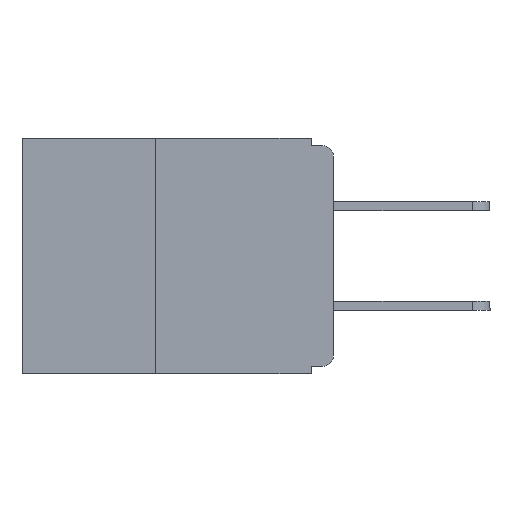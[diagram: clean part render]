
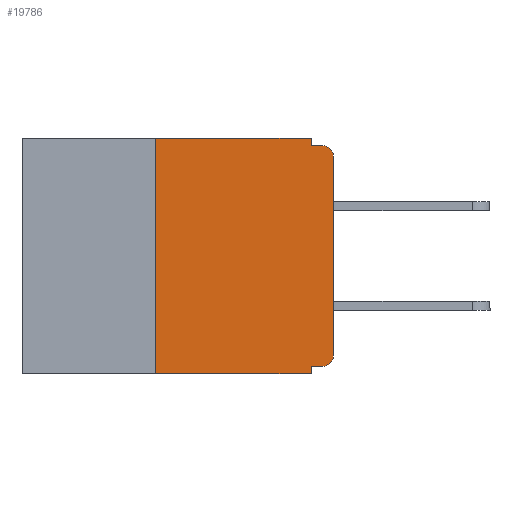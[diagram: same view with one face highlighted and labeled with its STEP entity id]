
A CAD part, left-side view. The second image highlights one B-rep face of the part: STEP entity #19786.
In plain terms, the highlighted planar face has unit normal (-1, 0, 0).
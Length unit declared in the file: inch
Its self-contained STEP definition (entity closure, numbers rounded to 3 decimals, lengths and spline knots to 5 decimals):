
#32 = CARTESIAN_POINT ( 'NONE',  ( 0., 0.031, -0.33 ) ) ;
#624 = VERTEX_POINT ( 'NONE', #32 ) ;
#645 = VERTEX_POINT ( 'NONE', #4479 ) ;
#825 = CARTESIAN_POINT ( 'NONE',  ( 0., 0.031, 0. ) ) ;
#1121 = VECTOR ( 'NONE', #8629, 39.37008 ) ;
#1186 = DIRECTION ( 'NONE',  ( 0., 0., 1. ) ) ;
#1564 = EDGE_CURVE ( 'NONE', #7581, #8345, #25323, .T. ) ;
#2440 = CARTESIAN_POINT ( 'NONE',  ( 0., 0., -0.01 ) ) ;
#2528 = ORIENTED_EDGE ( 'NONE', *, *, #4755, .T. ) ;
#3436 = LINE ( 'NONE', #8427, #21865 ) ;
#3734 = CIRCLE ( 'NONE', #17388, 0.015 ) ;
#4479 = CARTESIAN_POINT ( 'NONE',  ( 0., 0.25, -0.33 ) ) ;
#4483 = VERTEX_POINT ( 'NONE', #14346 ) ;
#4755 = EDGE_CURVE ( 'NONE', #22845, #7918, #9734, .T. ) ;
#4985 = DIRECTION ( 'NONE',  ( 0., -1., 0. ) ) ;
#6077 = VERTEX_POINT ( 'NONE', #9265 ) ;
#6265 = LINE ( 'NONE', #22654, #18276 ) ;
#7231 = CARTESIAN_POINT ( 'NONE',  ( 0., 0.015, -0.305 ) ) ;
#7581 = VERTEX_POINT ( 'NONE', #825 ) ;
#7740 = LINE ( 'NONE', #25043, #1121 ) ;
#7918 = VERTEX_POINT ( 'NONE', #28722 ) ;
#7936 = VECTOR ( 'NONE', #21931, 39.37008 ) ;
#8121 = ORIENTED_EDGE ( 'NONE', *, *, #26197, .T. ) ;
#8345 = VERTEX_POINT ( 'NONE', #16468 ) ;
#8427 = CARTESIAN_POINT ( 'NONE',  ( 0., 0., 0. ) ) ;
#8629 = DIRECTION ( 'NONE',  ( 0., -1., 0. ) ) ;
#9265 = CARTESIAN_POINT ( 'NONE',  ( 0., 0.031, -0.32 ) ) ;
#9291 = DIRECTION ( 'NONE',  ( 0., 1., 0. ) ) ;
#9700 = EDGE_CURVE ( 'NONE', #29924, #6077, #18430, .T. ) ;
#9725 = DIRECTION ( 'NONE',  ( 0., 0., -1. ) ) ;
#9734 = CIRCLE ( 'NONE', #17256, 0.015 ) ;
#9799 = CARTESIAN_POINT ( 'NONE',  ( 0., 0., -0.025 ) ) ;
#10445 = DIRECTION ( 'NONE',  ( 1., 0., 0. ) ) ;
#12741 = PLANE ( 'NONE',  #28231 ) ;
#14346 = CARTESIAN_POINT ( 'NONE',  ( 0., 0., -0.305 ) ) ;
#14945 = CARTESIAN_POINT ( 'NONE',  ( 0., 0.015, -0.32 ) ) ;
#15527 = DIRECTION ( 'NONE',  ( 0., 0., -1. ) ) ;
#15564 = DIRECTION ( 'NONE',  ( -1., 0., 0. ) ) ;
#15956 = CARTESIAN_POINT ( 'NONE',  ( 0., 0.015, -0.025 ) ) ;
#16377 = CARTESIAN_POINT ( 'NONE',  ( 0., 0., -0.32 ) ) ;
#16468 = CARTESIAN_POINT ( 'NONE',  ( 0., 0.031, -0.01 ) ) ;
#16560 = CARTESIAN_POINT ( 'NONE',  ( 0., 0.25, 0. ) ) ;
#16858 = ORIENTED_EDGE ( 'NONE', *, *, #17650, .F. ) ;
#16893 = EDGE_LOOP ( 'NONE', ( #18724, #2528, #16858, #24635, #30040, #24900, #8121, #21012, #29173, #21923 ) ) ;
#17256 = AXIS2_PLACEMENT_3D ( 'NONE', #15956, #15564, #15527 ) ;
#17388 = AXIS2_PLACEMENT_3D ( 'NONE', #7231, #23844, #9725 ) ;
#17467 = FACE_OUTER_BOUND ( 'NONE', #16893, .T. ) ;
#17650 = EDGE_CURVE ( 'NONE', #8345, #7918, #19851, .T. ) ;
#18276 = VECTOR ( 'NONE', #24957, 39.37008 ) ;
#18430 = LINE ( 'NONE', #16377, #29887 ) ;
#18719 = CARTESIAN_POINT ( 'NONE',  ( 0., 0.031, 0. ) ) ;
#18724 = ORIENTED_EDGE ( 'NONE', *, *, #26974, .T. ) ;
#19109 = VECTOR ( 'NONE', #4985, 39.37008 ) ;
#19264 = EDGE_CURVE ( 'NONE', #19511, #7581, #6265, .T. ) ;
#19511 = VERTEX_POINT ( 'NONE', #16560 ) ;
#19786 = ADVANCED_FACE ( 'NONE', ( #17467 ), #12741, .F. ) ;
#19851 = LINE ( 'NONE', #2440, #19109 ) ;
#21012 = ORIENTED_EDGE ( 'NONE', *, *, #24658, .F. ) ;
#21316 = VECTOR ( 'NONE', #1186, 39.37008 ) ;
#21865 = VECTOR ( 'NONE', #22664, 39.37008 ) ;
#21923 = ORIENTED_EDGE ( 'NONE', *, *, #29037, .T. ) ;
#21931 = DIRECTION ( 'NONE',  ( 0., 0., -1. ) ) ;
#22654 = CARTESIAN_POINT ( 'NONE',  ( 0., 0.437, 0. ) ) ;
#22664 = DIRECTION ( 'NONE',  ( 0., 0., 1. ) ) ;
#22845 = VERTEX_POINT ( 'NONE', #9799 ) ;
#23844 = DIRECTION ( 'NONE',  ( -1., 0., 0. ) ) ;
#24507 = CARTESIAN_POINT ( 'NONE',  ( 0., 0.437, 0. ) ) ;
#24635 = ORIENTED_EDGE ( 'NONE', *, *, #1564, .F. ) ;
#24658 = EDGE_CURVE ( 'NONE', #6077, #624, #25801, .T. ) ;
#24900 = ORIENTED_EDGE ( 'NONE', *, *, #30715, .F. ) ;
#24957 = DIRECTION ( 'NONE',  ( 0., -1., 0. ) ) ;
#25043 = CARTESIAN_POINT ( 'NONE',  ( 0., 0.437, -0.33 ) ) ;
#25089 = VECTOR ( 'NONE', #28177, 39.37008 ) ;
#25323 = LINE ( 'NONE', #18719, #7936 ) ;
#25801 = LINE ( 'NONE', #25926, #25089 ) ;
#25926 = CARTESIAN_POINT ( 'NONE',  ( 0., 0.031, -0.33 ) ) ;
#26197 = EDGE_CURVE ( 'NONE', #645, #624, #7740, .T. ) ;
#26794 = DIRECTION ( 'NONE',  ( 0., 0., -1. ) ) ;
#26974 = EDGE_CURVE ( 'NONE', #4483, #22845, #3436, .T. ) ;
#27360 = LINE ( 'NONE', #29620, #21316 ) ;
#28177 = DIRECTION ( 'NONE',  ( 0., 0., -1. ) ) ;
#28231 = AXIS2_PLACEMENT_3D ( 'NONE', #24507, #10445, #26794 ) ;
#28722 = CARTESIAN_POINT ( 'NONE',  ( 0., 0.015, -0.01 ) ) ;
#29037 = EDGE_CURVE ( 'NONE', #29924, #4483, #3734, .T. ) ;
#29173 = ORIENTED_EDGE ( 'NONE', *, *, #9700, .F. ) ;
#29620 = CARTESIAN_POINT ( 'NONE',  ( 0., 0.25, -0.33 ) ) ;
#29887 = VECTOR ( 'NONE', #9291, 39.37008 ) ;
#29924 = VERTEX_POINT ( 'NONE', #14945 ) ;
#30040 = ORIENTED_EDGE ( 'NONE', *, *, #19264, .F. ) ;
#30715 = EDGE_CURVE ( 'NONE', #645, #19511, #27360, .T. ) ;
